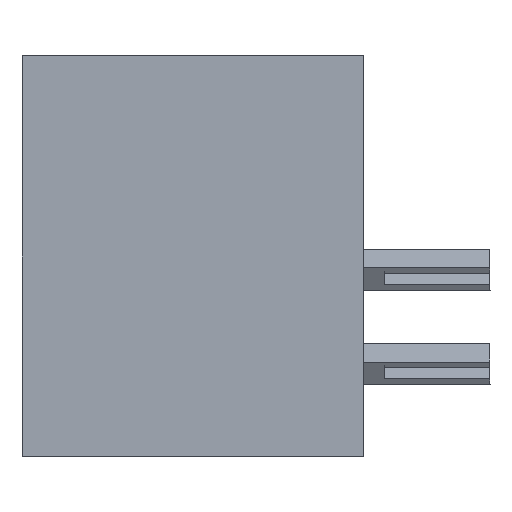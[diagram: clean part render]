
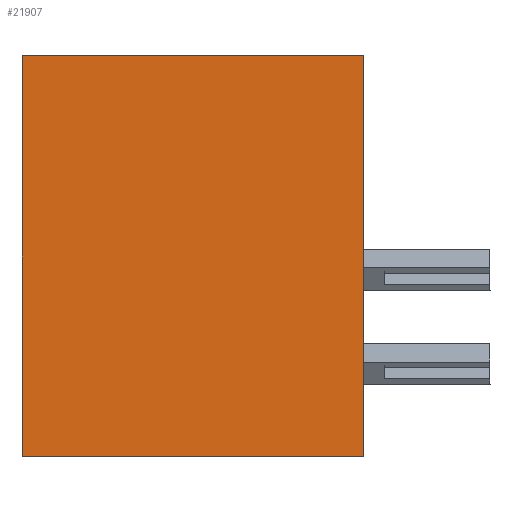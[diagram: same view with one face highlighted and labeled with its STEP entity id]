
A CAD part, left-side view. The second image highlights one B-rep face of the part: STEP entity #21907.
In plain terms, the highlighted planar face has unit normal (-1, 0, 0).
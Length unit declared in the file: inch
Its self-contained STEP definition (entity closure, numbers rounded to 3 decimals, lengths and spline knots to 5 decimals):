
#208 = ORIENTED_EDGE ( 'NONE', *, *, #3214, .F. ) ;
#1029 = LINE ( 'NONE', #12616, #15925 ) ;
#1237 = VERTEX_POINT ( 'NONE', #16827 ) ;
#2515 = LINE ( 'NONE', #20237, #21870 ) ;
#3117 = DIRECTION ( 'NONE',  ( 0., 0., 1. ) ) ;
#3214 = EDGE_CURVE ( 'NONE', #4303, #18003, #21763, .T. ) ;
#3484 = CARTESIAN_POINT ( 'NONE',  ( 0., 0., -0.531 ) ) ;
#3625 = FACE_OUTER_BOUND ( 'NONE', #10575, .T. ) ;
#4303 = VERTEX_POINT ( 'NONE', #22315 ) ;
#4564 = EDGE_CURVE ( 'NONE', #18003, #1237, #11096, .T. ) ;
#4685 = CARTESIAN_POINT ( 'NONE',  ( 0., 0.453, 0. ) ) ;
#6515 = PLANE ( 'NONE',  #11676 ) ;
#10413 = EDGE_CURVE ( 'NONE', #4303, #14417, #1029, .T. ) ;
#10575 = EDGE_LOOP ( 'NONE', ( #22082, #18579, #208, #21892 ) ) ;
#11096 = LINE ( 'NONE', #17187, #13007 ) ;
#11676 = AXIS2_PLACEMENT_3D ( 'NONE', #4685, #22364, #19031 ) ;
#12032 = DIRECTION ( 'NONE',  ( 0., -1., 0. ) ) ;
#12392 = DIRECTION ( 'NONE',  ( 0., -1., 0. ) ) ;
#12616 = CARTESIAN_POINT ( 'NONE',  ( 0., 0.453, -0.531 ) ) ;
#13007 = VECTOR ( 'NONE', #12032, 39.37008 ) ;
#13258 = DIRECTION ( 'NONE',  ( 0., 0., 1. ) ) ;
#13769 = CARTESIAN_POINT ( 'NONE',  ( 0., 0.453, 0. ) ) ;
#14417 = VERTEX_POINT ( 'NONE', #3484 ) ;
#15925 = VECTOR ( 'NONE', #12392, 39.37008 ) ;
#16501 = EDGE_CURVE ( 'NONE', #14417, #1237, #2515, .T. ) ;
#16827 = CARTESIAN_POINT ( 'NONE',  ( 0., 0., 0. ) ) ;
#17061 = VECTOR ( 'NONE', #3117, 39.37008 ) ;
#17187 = CARTESIAN_POINT ( 'NONE',  ( 0., 0.453, 0. ) ) ;
#17567 = CARTESIAN_POINT ( 'NONE',  ( 0., 0.453, 0. ) ) ;
#18003 = VERTEX_POINT ( 'NONE', #17567 ) ;
#18579 = ORIENTED_EDGE ( 'NONE', *, *, #4564, .F. ) ;
#19031 = DIRECTION ( 'NONE',  ( 0., 0., -1. ) ) ;
#20237 = CARTESIAN_POINT ( 'NONE',  ( 0., 0., 0. ) ) ;
#21763 = LINE ( 'NONE', #13769, #17061 ) ;
#21870 = VECTOR ( 'NONE', #13258, 39.37008 ) ;
#21892 = ORIENTED_EDGE ( 'NONE', *, *, #10413, .T. ) ;
#21907 = ADVANCED_FACE ( 'NONE', ( #3625 ), #6515, .F. ) ;
#22082 = ORIENTED_EDGE ( 'NONE', *, *, #16501, .T. ) ;
#22315 = CARTESIAN_POINT ( 'NONE',  ( 0., 0.453, -0.531 ) ) ;
#22364 = DIRECTION ( 'NONE',  ( 1., 0., 0. ) ) ;
